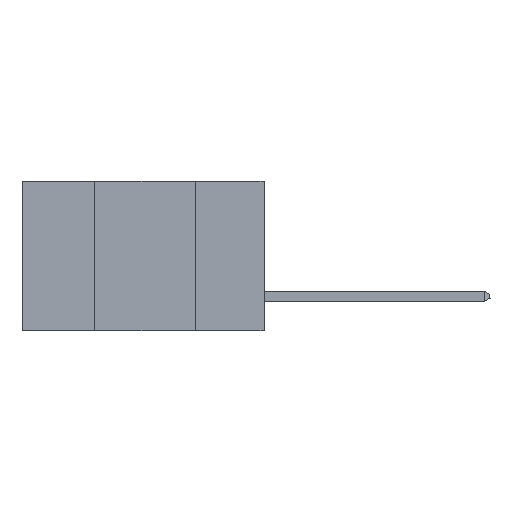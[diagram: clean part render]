
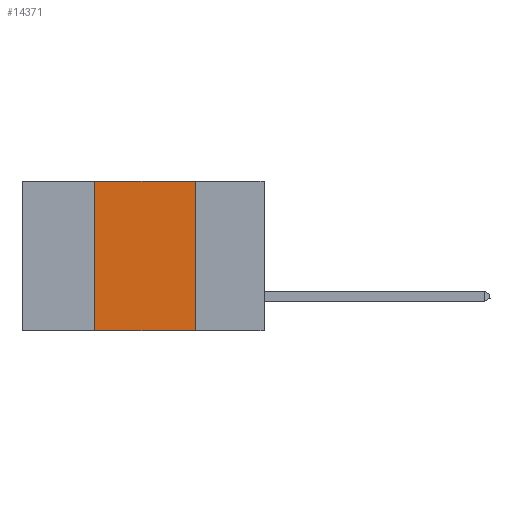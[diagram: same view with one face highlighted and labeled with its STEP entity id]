
A CAD part, left-side view. The second image highlights one B-rep face of the part: STEP entity #14371.
In plain terms, the highlighted planar face has unit normal (-1, 0, 0).
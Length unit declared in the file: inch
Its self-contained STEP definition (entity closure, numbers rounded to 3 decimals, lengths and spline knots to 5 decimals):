
#223 = DIRECTION ( 'NONE',  ( 0., 0., -1. ) ) ;
#428 = AXIS2_PLACEMENT_3D ( 'NONE', #18540, #20101, #10149 ) ;
#734 = CARTESIAN_POINT ( 'NONE',  ( 0., 0.42, 0. ) ) ;
#879 = VECTOR ( 'NONE', #223, 39.37008 ) ;
#1262 = VECTOR ( 'NONE', #3680, 39.37008 ) ;
#1584 = PLANE ( 'NONE',  #428 ) ;
#2425 = DIRECTION ( 'NONE',  ( 0., 0., 1. ) ) ;
#3130 = LINE ( 'NONE', #6967, #1262 ) ;
#3403 = VERTEX_POINT ( 'NONE', #9180 ) ;
#3680 = DIRECTION ( 'NONE',  ( 0., -1., 0. ) ) ;
#4134 = ORIENTED_EDGE ( 'NONE', *, *, #12585, .T. ) ;
#4227 = EDGE_CURVE ( 'NONE', #13161, #3403, #7531, .T. ) ;
#4295 = VERTEX_POINT ( 'NONE', #12752 ) ;
#4862 = CARTESIAN_POINT ( 'NONE',  ( 0., 0.17, 0. ) ) ;
#5571 = CARTESIAN_POINT ( 'NONE',  ( 0., 0.17, 0. ) ) ;
#5585 = ORIENTED_EDGE ( 'NONE', *, *, #8163, .F. ) ;
#6500 = VERTEX_POINT ( 'NONE', #9174 ) ;
#6967 = CARTESIAN_POINT ( 'NONE',  ( 0., 0.6, 0. ) ) ;
#7531 = LINE ( 'NONE', #5571, #879 ) ;
#7797 = EDGE_CURVE ( 'NONE', #6500, #4295, #14656, .T. ) ;
#8163 = EDGE_CURVE ( 'NONE', #4295, #13161, #3130, .T. ) ;
#8343 = ORIENTED_EDGE ( 'NONE', *, *, #4227, .F. ) ;
#9174 = CARTESIAN_POINT ( 'NONE',  ( 0., 0.42, -0.37 ) ) ;
#9180 = CARTESIAN_POINT ( 'NONE',  ( 0., 0.17, -0.37 ) ) ;
#10149 = DIRECTION ( 'NONE',  ( 0., 0., -1. ) ) ;
#10891 = DIRECTION ( 'NONE',  ( 0., -1., 0. ) ) ;
#12526 = LINE ( 'NONE', #12536, #20804 ) ;
#12536 = CARTESIAN_POINT ( 'NONE',  ( 0., 0.6, -0.37 ) ) ;
#12585 = EDGE_CURVE ( 'NONE', #6500, #3403, #12526, .T. ) ;
#12614 = EDGE_LOOP ( 'NONE', ( #8343, #5585, #15278, #4134 ) ) ;
#12752 = CARTESIAN_POINT ( 'NONE',  ( 0., 0.42, 0. ) ) ;
#13161 = VERTEX_POINT ( 'NONE', #4862 ) ;
#14371 = ADVANCED_FACE ( 'NONE', ( #15289 ), #1584, .F. ) ;
#14656 = LINE ( 'NONE', #734, #19455 ) ;
#15278 = ORIENTED_EDGE ( 'NONE', *, *, #7797, .F. ) ;
#15289 = FACE_OUTER_BOUND ( 'NONE', #12614, .T. ) ;
#18540 = CARTESIAN_POINT ( 'NONE',  ( 0., 0.6, 0. ) ) ;
#19455 = VECTOR ( 'NONE', #2425, 39.37008 ) ;
#20101 = DIRECTION ( 'NONE',  ( 1., 0., 0. ) ) ;
#20804 = VECTOR ( 'NONE', #10891, 39.37008 ) ;
